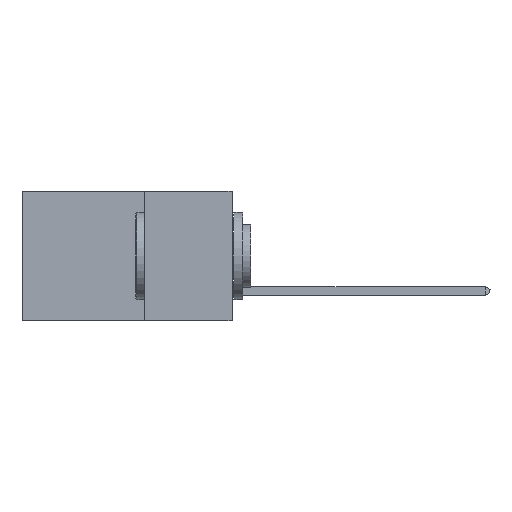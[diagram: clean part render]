
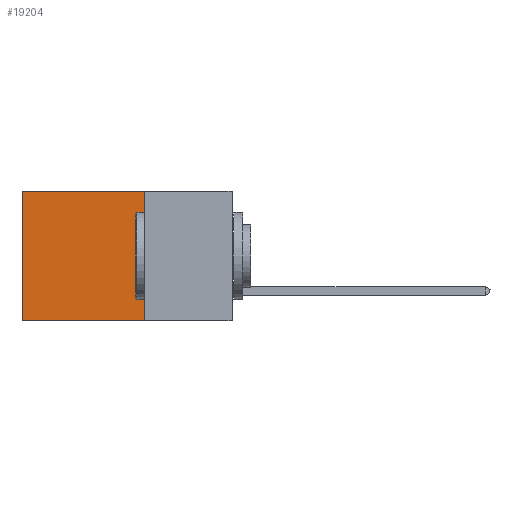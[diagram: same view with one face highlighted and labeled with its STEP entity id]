
A CAD part, left-side view. The second image highlights one B-rep face of the part: STEP entity #19204.
In plain terms, the highlighted planar face has unit normal (-1, 0, 0).
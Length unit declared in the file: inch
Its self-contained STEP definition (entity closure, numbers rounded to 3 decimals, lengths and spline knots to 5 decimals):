
#3940 = VERTEX_POINT ( 'NONE', #5538 ) ;
#4307 = EDGE_CURVE ( 'NONE', #3940, #27471, #23160, .T. ) ;
#4709 = CARTESIAN_POINT ( 'NONE',  ( 0.2875, 0.6, -0.37 ) ) ;
#5538 = CARTESIAN_POINT ( 'NONE',  ( 0.2875, 0.25, 0. ) ) ;
#6047 = VERTEX_POINT ( 'NONE', #28256 ) ;
#8600 = VECTOR ( 'NONE', #38426, 39.37008 ) ;
#9876 = CARTESIAN_POINT ( 'NONE',  ( 0.2875, 0.25, 0. ) ) ;
#10266 = PLANE ( 'NONE',  #21400 ) ;
#11503 = VECTOR ( 'NONE', #33254, 39.37008 ) ;
#13169 = CARTESIAN_POINT ( 'NONE',  ( 0.2875, 0.6, 0. ) ) ;
#14368 = CARTESIAN_POINT ( 'NONE',  ( 0.2875, 0.25, 0. ) ) ;
#15763 = DIRECTION ( 'NONE',  ( 0., 0., -1. ) ) ;
#16394 = ORIENTED_EDGE ( 'NONE', *, *, #42707, .F. ) ;
#18005 = ORIENTED_EDGE ( 'NONE', *, *, #23368, .T. ) ;
#18656 = DIRECTION ( 'NONE',  ( 1., 0., 0. ) ) ;
#19204 = ADVANCED_FACE ( 'NONE', ( #39917 ), #10266, .F. ) ;
#21400 = AXIS2_PLACEMENT_3D ( 'NONE', #14368, #18656, #25815 ) ;
#23160 = LINE ( 'NONE', #34242, #50604 ) ;
#23361 = ORIENTED_EDGE ( 'NONE', *, *, #45499, .T. ) ;
#23368 = EDGE_CURVE ( 'NONE', #3940, #6047, #45664, .T. ) ;
#24472 = LINE ( 'NONE', #46255, #8600 ) ;
#25815 = DIRECTION ( 'NONE',  ( 0., 0., -1. ) ) ;
#26647 = VECTOR ( 'NONE', #15763, 39.37008 ) ;
#27471 = VERTEX_POINT ( 'NONE', #33645 ) ;
#28256 = CARTESIAN_POINT ( 'NONE',  ( 0.2875, 0.6, 0. ) ) ;
#29509 = VERTEX_POINT ( 'NONE', #4709 ) ;
#31980 = EDGE_LOOP ( 'NONE', ( #23361, #16394, #44793, #18005 ) ) ;
#32418 = DIRECTION ( 'NONE',  ( 0., 0., -1. ) ) ;
#33254 = DIRECTION ( 'NONE',  ( 0., 1., 0. ) ) ;
#33645 = CARTESIAN_POINT ( 'NONE',  ( 0.2875, 0.25, -0.37 ) ) ;
#34242 = CARTESIAN_POINT ( 'NONE',  ( 0.2875, 0.25, 0. ) ) ;
#37598 = LINE ( 'NONE', #13169, #26647 ) ;
#38426 = DIRECTION ( 'NONE',  ( 0., 1., 0. ) ) ;
#39917 = FACE_OUTER_BOUND ( 'NONE', #31980, .T. ) ;
#42707 = EDGE_CURVE ( 'NONE', #27471, #29509, #24472, .T. ) ;
#44793 = ORIENTED_EDGE ( 'NONE', *, *, #4307, .F. ) ;
#45499 = EDGE_CURVE ( 'NONE', #6047, #29509, #37598, .T. ) ;
#45664 = LINE ( 'NONE', #9876, #11503 ) ;
#46255 = CARTESIAN_POINT ( 'NONE',  ( 0.2875, 0.25, -0.37 ) ) ;
#50604 = VECTOR ( 'NONE', #32418, 39.37008 ) ;
